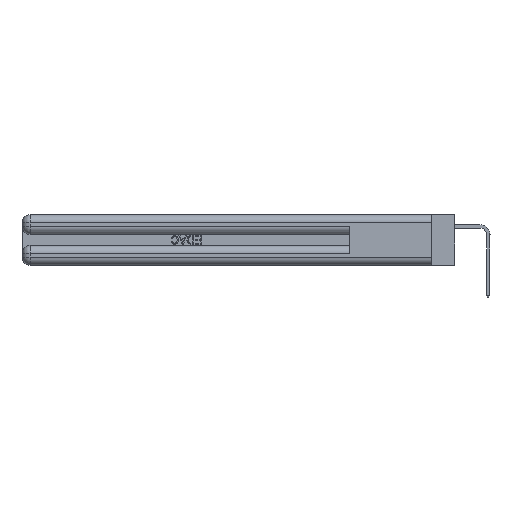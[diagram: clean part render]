
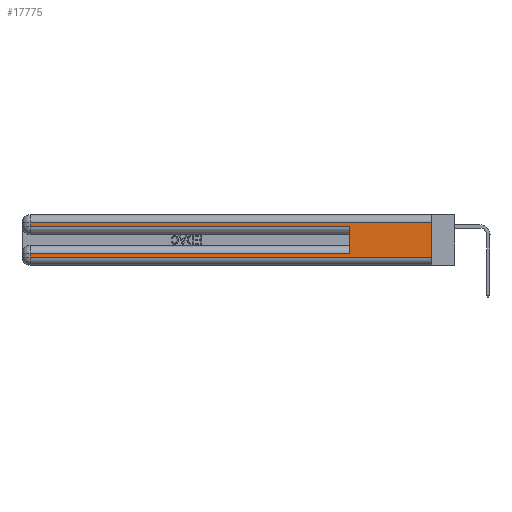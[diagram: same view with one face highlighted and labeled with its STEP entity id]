
A CAD part, left-side view. The second image highlights one B-rep face of the part: STEP entity #17775.
In plain terms, the highlighted planar face has unit normal (-1, 0, 0).
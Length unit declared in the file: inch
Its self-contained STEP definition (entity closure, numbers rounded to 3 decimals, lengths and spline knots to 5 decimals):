
#926 = EDGE_CURVE ( 'NONE', #30671, #11512, #19383, .T. ) ;
#1261 = CARTESIAN_POINT ( 'NONE',  ( 0., 2.94, 0.085 ) ) ;
#2412 = ORIENTED_EDGE ( 'NONE', *, *, #926, .F. ) ;
#2952 = CARTESIAN_POINT ( 'NONE',  ( 0., 0., 0.285 ) ) ;
#3020 = ORIENTED_EDGE ( 'NONE', *, *, #9021, .T. ) ;
#3388 = DIRECTION ( 'NONE',  ( 0., 0., -1. ) ) ;
#4013 = VECTOR ( 'NONE', #13447, 39.37008 ) ;
#6990 = CARTESIAN_POINT ( 'NONE',  ( 0., 2.94, 0.37 ) ) ;
#7063 = LINE ( 'NONE', #2952, #36318 ) ;
#7314 = PLANE ( 'NONE',  #21944 ) ;
#7897 = CARTESIAN_POINT ( 'NONE',  ( 0., 0.6, 0.085 ) ) ;
#8009 = CARTESIAN_POINT ( 'NONE',  ( 0., 0., 0.085 ) ) ;
#9021 = EDGE_CURVE ( 'NONE', #49225, #18225, #16424, .T. ) ;
#9087 = VECTOR ( 'NONE', #31510, 39.37008 ) ;
#9549 = CARTESIAN_POINT ( 'NONE',  ( 0., 0., 0.31 ) ) ;
#9638 = ORIENTED_EDGE ( 'NONE', *, *, #44567, .T. ) ;
#10375 = CARTESIAN_POINT ( 'NONE',  ( 0., 0., 0.06 ) ) ;
#11161 = DIRECTION ( 'NONE',  ( 1., 0., 0. ) ) ;
#11464 = VECTOR ( 'NONE', #20262, 39.37008 ) ;
#11512 = VERTEX_POINT ( 'NONE', #14003 ) ;
#12163 = EDGE_CURVE ( 'NONE', #21178, #30937, #7063, .T. ) ;
#12258 = CARTESIAN_POINT ( 'NONE',  ( 0., 0., 0.37 ) ) ;
#12405 = EDGE_CURVE ( 'NONE', #46276, #49225, #45846, .T. ) ;
#12682 = CARTESIAN_POINT ( 'NONE',  ( 0., 2.94, 0.285 ) ) ;
#13134 = VECTOR ( 'NONE', #3388, 39.37008 ) ;
#13447 = DIRECTION ( 'NONE',  ( 0., 1., 0. ) ) ;
#14003 = CARTESIAN_POINT ( 'NONE',  ( 0., 0., 0.06 ) ) ;
#15725 = CARTESIAN_POINT ( 'NONE',  ( 0., 0., 0.31 ) ) ;
#16395 = CARTESIAN_POINT ( 'NONE',  ( 0., 0.6, 0.145 ) ) ;
#16424 = LINE ( 'NONE', #48749, #47932 ) ;
#16527 = VERTEX_POINT ( 'NONE', #41304 ) ;
#16803 = LINE ( 'NONE', #6990, #13134 ) ;
#17110 = ORIENTED_EDGE ( 'NONE', *, *, #20413, .F. ) ;
#17775 = ADVANCED_FACE ( 'NONE', ( #19884 ), #7314, .F. ) ;
#18225 = VERTEX_POINT ( 'NONE', #24272 ) ;
#18323 = DIRECTION ( 'NONE',  ( 0., -1., 0. ) ) ;
#18450 = CARTESIAN_POINT ( 'NONE',  ( 0., 0., 0.37 ) ) ;
#18568 = EDGE_CURVE ( 'NONE', #16527, #21178, #16803, .T. ) ;
#19383 = LINE ( 'NONE', #12258, #9087 ) ;
#19884 = FACE_OUTER_BOUND ( 'NONE', #34849, .T. ) ;
#20262 = DIRECTION ( 'NONE',  ( 0., 0., 1. ) ) ;
#20413 = EDGE_CURVE ( 'NONE', #46276, #30937, #33012, .T. ) ;
#21178 = VERTEX_POINT ( 'NONE', #12682 ) ;
#21944 = AXIS2_PLACEMENT_3D ( 'NONE', #18450, #11161, #37854 ) ;
#22690 = EDGE_CURVE ( 'NONE', #18225, #11512, #47020, .T. ) ;
#24272 = CARTESIAN_POINT ( 'NONE',  ( 0., 2.94, 0.06 ) ) ;
#26014 = DIRECTION ( 'NONE',  ( 0., 0., -1. ) ) ;
#30671 = VERTEX_POINT ( 'NONE', #15725 ) ;
#30937 = VERTEX_POINT ( 'NONE', #32524 ) ;
#30979 = DIRECTION ( 'NONE',  ( 0., 1., 0. ) ) ;
#31510 = DIRECTION ( 'NONE',  ( 0., 0., -1. ) ) ;
#31564 = ORIENTED_EDGE ( 'NONE', *, *, #18568, .T. ) ;
#32524 = CARTESIAN_POINT ( 'NONE',  ( 0., 0.6, 0.285 ) ) ;
#33012 = LINE ( 'NONE', #16395, #11464 ) ;
#33981 = ORIENTED_EDGE ( 'NONE', *, *, #12405, .T. ) ;
#34849 = EDGE_LOOP ( 'NONE', ( #2412, #9638, #31564, #34966, #17110, #33981, #3020, #39444 ) ) ;
#34966 = ORIENTED_EDGE ( 'NONE', *, *, #12163, .T. ) ;
#35709 = VECTOR ( 'NONE', #18323, 39.37008 ) ;
#36318 = VECTOR ( 'NONE', #48560, 39.37008 ) ;
#37854 = DIRECTION ( 'NONE',  ( 0., 0., -1. ) ) ;
#39444 = ORIENTED_EDGE ( 'NONE', *, *, #22690, .T. ) ;
#41304 = CARTESIAN_POINT ( 'NONE',  ( 0., 2.94, 0.31 ) ) ;
#42123 = LINE ( 'NONE', #9549, #4013 ) ;
#44567 = EDGE_CURVE ( 'NONE', #30671, #16527, #42123, .T. ) ;
#44646 = VECTOR ( 'NONE', #30979, 39.37008 ) ;
#45846 = LINE ( 'NONE', #8009, #44646 ) ;
#46276 = VERTEX_POINT ( 'NONE', #7897 ) ;
#47020 = LINE ( 'NONE', #10375, #35709 ) ;
#47932 = VECTOR ( 'NONE', #26014, 39.37008 ) ;
#48560 = DIRECTION ( 'NONE',  ( 0., -1., 0. ) ) ;
#48749 = CARTESIAN_POINT ( 'NONE',  ( 0., 2.94, 0.37 ) ) ;
#49225 = VERTEX_POINT ( 'NONE', #1261 ) ;
